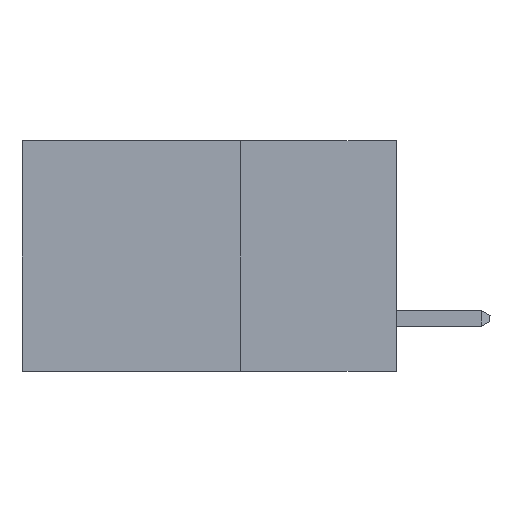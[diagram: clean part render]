
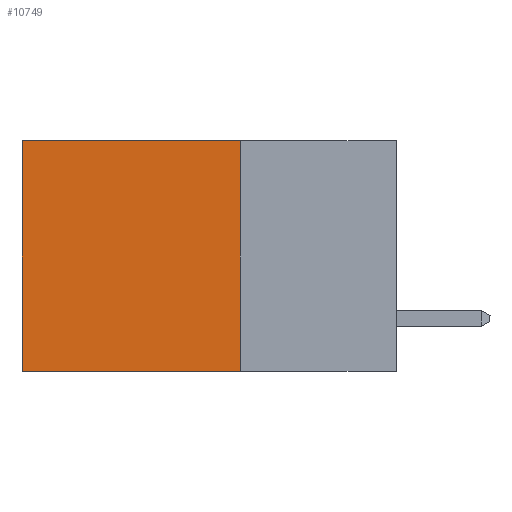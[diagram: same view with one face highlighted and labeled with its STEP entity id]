
A CAD part, left-side view. The second image highlights one B-rep face of the part: STEP entity #10749.
In plain terms, the highlighted planar face has unit normal (-1, 0, 0).
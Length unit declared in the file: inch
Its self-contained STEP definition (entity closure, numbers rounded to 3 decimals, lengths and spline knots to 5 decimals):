
#309 = ORIENTED_EDGE ( 'NONE', *, *, #7647, .F. ) ;
#760 = VERTEX_POINT ( 'NONE', #17444 ) ;
#807 = CARTESIAN_POINT ( 'NONE',  ( 0.2615, 0.6, -0.37 ) ) ;
#2152 = LINE ( 'NONE', #807, #12106 ) ;
#2890 = LINE ( 'NONE', #14119, #8217 ) ;
#3727 = ORIENTED_EDGE ( 'NONE', *, *, #16307, .T. ) ;
#3760 = DIRECTION ( 'NONE',  ( 1., 0., 0. ) ) ;
#4044 = LINE ( 'NONE', #6656, #7725 ) ;
#4046 = EDGE_CURVE ( 'NONE', #760, #9932, #2152, .T. ) ;
#4218 = CARTESIAN_POINT ( 'NONE',  ( 0.2615, 0.25, 0. ) ) ;
#5085 = CARTESIAN_POINT ( 'NONE',  ( 0.2615, 0.6, -0.37 ) ) ;
#5183 = CARTESIAN_POINT ( 'NONE',  ( 0.2615, 0.25, -0.37 ) ) ;
#5855 = DIRECTION ( 'NONE',  ( 0., 1., 0. ) ) ;
#5863 = DIRECTION ( 'NONE',  ( 0., 0., -1. ) ) ;
#6656 = CARTESIAN_POINT ( 'NONE',  ( 0.2615, 0.25, 0. ) ) ;
#7366 = LINE ( 'NONE', #12840, #9836 ) ;
#7478 = EDGE_LOOP ( 'NONE', ( #11439, #309, #12405, #3727 ) ) ;
#7647 = EDGE_CURVE ( 'NONE', #8681, #9932, #7366, .T. ) ;
#7725 = VECTOR ( 'NONE', #8085, 39.37008 ) ;
#8085 = DIRECTION ( 'NONE',  ( 0., 1., 0. ) ) ;
#8217 = VECTOR ( 'NONE', #5863, 39.37008 ) ;
#8681 = VERTEX_POINT ( 'NONE', #5183 ) ;
#9836 = VECTOR ( 'NONE', #5855, 39.37008 ) ;
#9932 = VERTEX_POINT ( 'NONE', #5085 ) ;
#10570 = PLANE ( 'NONE',  #11065 ) ;
#10584 = EDGE_CURVE ( 'NONE', #16512, #8681, #2890, .T. ) ;
#10749 = ADVANCED_FACE ( 'NONE', ( #16060 ), #10570, .F. ) ;
#11065 = AXIS2_PLACEMENT_3D ( 'NONE', #13355, #3760, #13447 ) ;
#11439 = ORIENTED_EDGE ( 'NONE', *, *, #4046, .T. ) ;
#12106 = VECTOR ( 'NONE', #17240, 39.37008 ) ;
#12405 = ORIENTED_EDGE ( 'NONE', *, *, #10584, .F. ) ;
#12840 = CARTESIAN_POINT ( 'NONE',  ( 0.2615, 0.25, -0.37 ) ) ;
#13355 = CARTESIAN_POINT ( 'NONE',  ( 0.2615, 0.25, -0.37 ) ) ;
#13447 = DIRECTION ( 'NONE',  ( 0., 0., -1. ) ) ;
#14119 = CARTESIAN_POINT ( 'NONE',  ( 0.2615, 0.25, -0.37 ) ) ;
#16060 = FACE_OUTER_BOUND ( 'NONE', #7478, .T. ) ;
#16307 = EDGE_CURVE ( 'NONE', #16512, #760, #4044, .T. ) ;
#16512 = VERTEX_POINT ( 'NONE', #4218 ) ;
#17240 = DIRECTION ( 'NONE',  ( 0., 0., -1. ) ) ;
#17444 = CARTESIAN_POINT ( 'NONE',  ( 0.2615, 0.6, 0. ) ) ;
